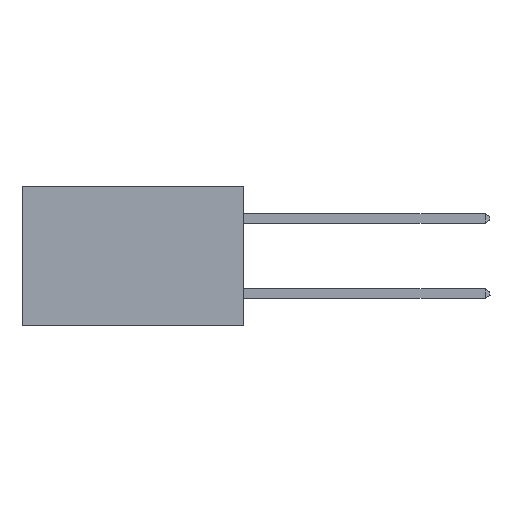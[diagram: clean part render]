
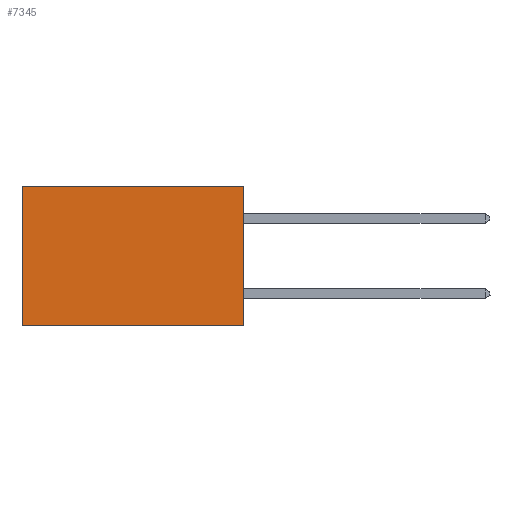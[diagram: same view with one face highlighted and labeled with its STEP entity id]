
A CAD part, left-side view. The second image highlights one B-rep face of the part: STEP entity #7345.
In plain terms, the highlighted planar face has unit normal (-1, 0, 0).
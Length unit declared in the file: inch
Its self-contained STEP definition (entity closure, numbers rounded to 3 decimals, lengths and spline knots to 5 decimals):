
#211 = CARTESIAN_POINT ( 'NONE',  ( 0.277, 0., -0.37 ) ) ;
#947 = CARTESIAN_POINT ( 'NONE',  ( 0.277, 0.59, -0.37 ) ) ;
#2412 = VECTOR ( 'NONE', #18374, 39.37008 ) ;
#2585 = ORIENTED_EDGE ( 'NONE', *, *, #22494, .T. ) ;
#5845 = FACE_OUTER_BOUND ( 'NONE', #8358, .T. ) ;
#7345 = ADVANCED_FACE ( 'NONE', ( #5845 ), #12972, .F. ) ;
#7473 = LINE ( 'NONE', #947, #21300 ) ;
#8358 = EDGE_LOOP ( 'NONE', ( #2585, #27683, #8963, #17103 ) ) ;
#8963 = ORIENTED_EDGE ( 'NONE', *, *, #18594, .F. ) ;
#9124 = LINE ( 'NONE', #11152, #15191 ) ;
#10397 = EDGE_CURVE ( 'NONE', #25832, #22295, #29112, .T. ) ;
#11152 = CARTESIAN_POINT ( 'NONE',  ( 0.277, 0., 0. ) ) ;
#12758 = DIRECTION ( 'NONE',  ( 0., 0., -1. ) ) ;
#12867 = DIRECTION ( 'NONE',  ( 1., 0., 0. ) ) ;
#12938 = CARTESIAN_POINT ( 'NONE',  ( 0.277, 0., -0.37 ) ) ;
#12972 = PLANE ( 'NONE',  #23033 ) ;
#13726 = DIRECTION ( 'NONE',  ( 0., 1., 0. ) ) ;
#15191 = VECTOR ( 'NONE', #13726, 39.37008 ) ;
#16050 = CARTESIAN_POINT ( 'NONE',  ( 0.277, 0., -0.37 ) ) ;
#16408 = DIRECTION ( 'NONE',  ( 0., 1., 0. ) ) ;
#17103 = ORIENTED_EDGE ( 'NONE', *, *, #22478, .T. ) ;
#18180 = VERTEX_POINT ( 'NONE', #32256 ) ;
#18374 = DIRECTION ( 'NONE',  ( 0., 0., -1. ) ) ;
#18594 = EDGE_CURVE ( 'NONE', #18180, #25832, #29109, .T. ) ;
#19114 = DIRECTION ( 'NONE',  ( 0., 0., -1. ) ) ;
#21300 = VECTOR ( 'NONE', #19114, 39.37008 ) ;
#21536 = VECTOR ( 'NONE', #16408, 39.37008 ) ;
#22295 = VERTEX_POINT ( 'NONE', #28530 ) ;
#22478 = EDGE_CURVE ( 'NONE', #18180, #23196, #9124, .T. ) ;
#22494 = EDGE_CURVE ( 'NONE', #23196, #22295, #7473, .T. ) ;
#23033 = AXIS2_PLACEMENT_3D ( 'NONE', #12938, #12867, #12758 ) ;
#23196 = VERTEX_POINT ( 'NONE', #29469 ) ;
#25832 = VERTEX_POINT ( 'NONE', #32034 ) ;
#27683 = ORIENTED_EDGE ( 'NONE', *, *, #10397, .F. ) ;
#28530 = CARTESIAN_POINT ( 'NONE',  ( 0.277, 0.59, -0.37 ) ) ;
#29109 = LINE ( 'NONE', #211, #2412 ) ;
#29112 = LINE ( 'NONE', #16050, #21536 ) ;
#29469 = CARTESIAN_POINT ( 'NONE',  ( 0.277, 0.59, 0. ) ) ;
#32034 = CARTESIAN_POINT ( 'NONE',  ( 0.277, 0., -0.37 ) ) ;
#32256 = CARTESIAN_POINT ( 'NONE',  ( 0.277, 0., 0. ) ) ;
